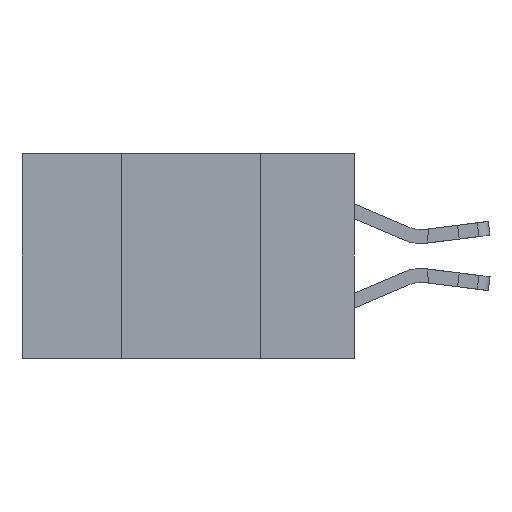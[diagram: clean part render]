
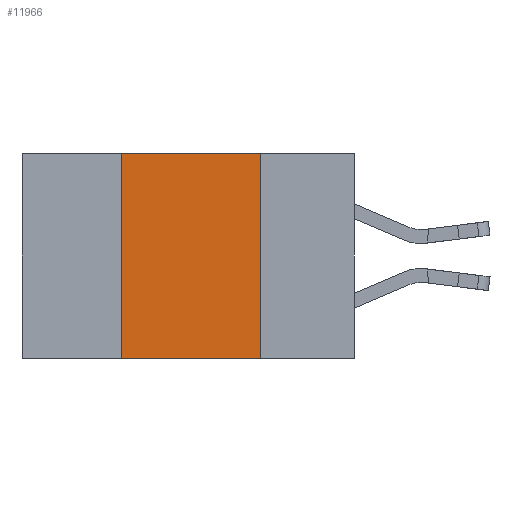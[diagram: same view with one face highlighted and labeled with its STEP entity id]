
A CAD part, left-side view. The second image highlights one B-rep face of the part: STEP entity #11966.
In plain terms, the highlighted planar face has unit normal (-1, 0, 0).
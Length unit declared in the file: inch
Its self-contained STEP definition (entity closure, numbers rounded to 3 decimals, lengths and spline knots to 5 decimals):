
#228 = VECTOR ( 'NONE', #10806, 39.37008 ) ;
#398 = LINE ( 'NONE', #7442, #10253 ) ;
#653 = LINE ( 'NONE', #4871, #5180 ) ;
#1196 = ORIENTED_EDGE ( 'NONE', *, *, #7830, .F. ) ;
#1349 = VERTEX_POINT ( 'NONE', #7298 ) ;
#1441 = DIRECTION ( 'NONE',  ( 0., 0., -1. ) ) ;
#1545 = PLANE ( 'NONE',  #10017 ) ;
#2655 = DIRECTION ( 'NONE',  ( 0., 0., 1. ) ) ;
#2716 = LINE ( 'NONE', #7250, #5269 ) ;
#3080 = CARTESIAN_POINT ( 'NONE',  ( 0., 0.17, 0. ) ) ;
#3262 = EDGE_CURVE ( 'NONE', #1349, #8288, #653, .T. ) ;
#3287 = VERTEX_POINT ( 'NONE', #9620 ) ;
#3556 = DIRECTION ( 'NONE',  ( 1., 0., 0. ) ) ;
#4237 = CARTESIAN_POINT ( 'NONE',  ( 0., 0.6, -0.37 ) ) ;
#4351 = ORIENTED_EDGE ( 'NONE', *, *, #8704, .F. ) ;
#4463 = ORIENTED_EDGE ( 'NONE', *, *, #10098, .T. ) ;
#4573 = EDGE_LOOP ( 'NONE', ( #1196, #6960, #4351, #4463 ) ) ;
#4871 = CARTESIAN_POINT ( 'NONE',  ( 0., 0.6, 0. ) ) ;
#5082 = LINE ( 'NONE', #4237, #228 ) ;
#5180 = VECTOR ( 'NONE', #11390, 39.37008 ) ;
#5269 = VECTOR ( 'NONE', #1441, 39.37008 ) ;
#6400 = FACE_OUTER_BOUND ( 'NONE', #4573, .T. ) ;
#6695 = CARTESIAN_POINT ( 'NONE',  ( 0., 0.17, -0.37 ) ) ;
#6960 = ORIENTED_EDGE ( 'NONE', *, *, #3262, .F. ) ;
#7250 = CARTESIAN_POINT ( 'NONE',  ( 0., 0.17, -0.37 ) ) ;
#7298 = CARTESIAN_POINT ( 'NONE',  ( 0., 0.42, 0. ) ) ;
#7442 = CARTESIAN_POINT ( 'NONE',  ( 0., 0.42, -0.37 ) ) ;
#7830 = EDGE_CURVE ( 'NONE', #8288, #8878, #2716, .T. ) ;
#8288 = VERTEX_POINT ( 'NONE', #3080 ) ;
#8704 = EDGE_CURVE ( 'NONE', #3287, #1349, #398, .T. ) ;
#8878 = VERTEX_POINT ( 'NONE', #6695 ) ;
#9266 = CARTESIAN_POINT ( 'NONE',  ( 0., 0.6, 0. ) ) ;
#9620 = CARTESIAN_POINT ( 'NONE',  ( 0., 0.42, -0.37 ) ) ;
#10017 = AXIS2_PLACEMENT_3D ( 'NONE', #9266, #3556, #10189 ) ;
#10098 = EDGE_CURVE ( 'NONE', #3287, #8878, #5082, .T. ) ;
#10189 = DIRECTION ( 'NONE',  ( 0., 0., -1. ) ) ;
#10253 = VECTOR ( 'NONE', #2655, 39.37008 ) ;
#10806 = DIRECTION ( 'NONE',  ( 0., -1., 0. ) ) ;
#11390 = DIRECTION ( 'NONE',  ( 0., -1., 0. ) ) ;
#11966 = ADVANCED_FACE ( 'NONE', ( #6400 ), #1545, .F. ) ;
